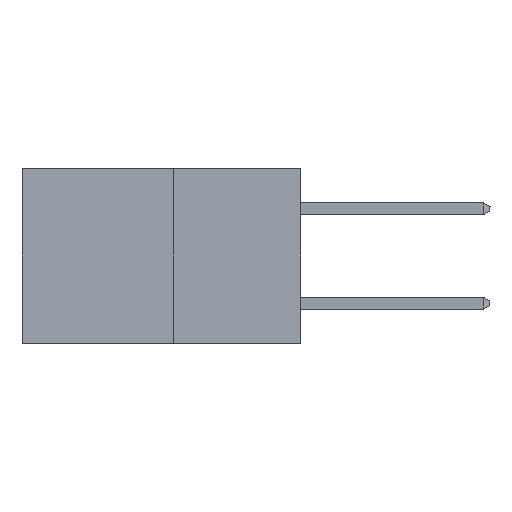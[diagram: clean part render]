
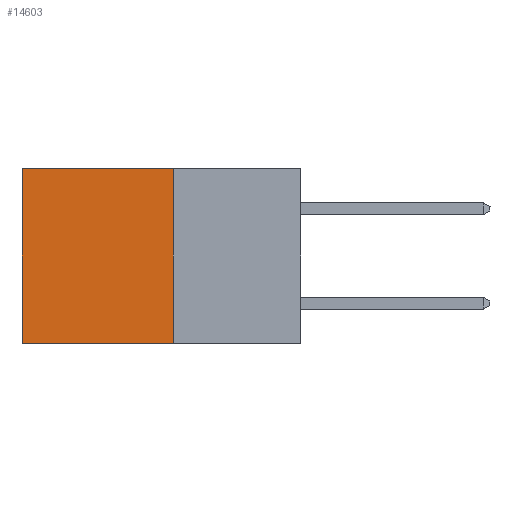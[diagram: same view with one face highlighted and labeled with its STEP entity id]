
A CAD part, left-side view. The second image highlights one B-rep face of the part: STEP entity #14603.
In plain terms, the highlighted planar face has unit normal (-1, 0, 0).
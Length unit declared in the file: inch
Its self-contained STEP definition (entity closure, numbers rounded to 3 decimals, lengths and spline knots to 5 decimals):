
#872 = CARTESIAN_POINT ( 'NONE',  ( 0.277, 0.27, 0. ) ) ;
#960 = VERTEX_POINT ( 'NONE', #5564 ) ;
#1803 = VERTEX_POINT ( 'NONE', #12594 ) ;
#2059 = CARTESIAN_POINT ( 'NONE',  ( 0.277, 0.59, -0.37 ) ) ;
#3305 = AXIS2_PLACEMENT_3D ( 'NONE', #14105, #4311, #14167 ) ;
#3553 = DIRECTION ( 'NONE',  ( 0., 0., -1. ) ) ;
#4311 = DIRECTION ( 'NONE',  ( 1., 0., 0. ) ) ;
#4386 = VECTOR ( 'NONE', #3553, 39.37008 ) ;
#4569 = EDGE_CURVE ( 'NONE', #16371, #11281, #10069, .T. ) ;
#5119 = DIRECTION ( 'NONE',  ( 0., 1., 0. ) ) ;
#5558 = ORIENTED_EDGE ( 'NONE', *, *, #14233, .F. ) ;
#5564 = CARTESIAN_POINT ( 'NONE',  ( 0.277, 0.27, -0.37 ) ) ;
#5967 = CARTESIAN_POINT ( 'NONE',  ( 0.277, 0.27, 0. ) ) ;
#6186 = DIRECTION ( 'NONE',  ( 0., 1., 0. ) ) ;
#6847 = VECTOR ( 'NONE', #5119, 39.37008 ) ;
#6970 = CARTESIAN_POINT ( 'NONE',  ( 0.277, 0.59, 0. ) ) ;
#7265 = LINE ( 'NONE', #16370, #6847 ) ;
#7583 = DIRECTION ( 'NONE',  ( 0., 0., -1. ) ) ;
#7658 = EDGE_CURVE ( 'NONE', #960, #1803, #7265, .T. ) ;
#8397 = ORIENTED_EDGE ( 'NONE', *, *, #7658, .F. ) ;
#8823 = EDGE_CURVE ( 'NONE', #11281, #1803, #17061, .T. ) ;
#9875 = PLANE ( 'NONE',  #3305 ) ;
#10009 = VECTOR ( 'NONE', #7583, 39.37008 ) ;
#10069 = LINE ( 'NONE', #5967, #10524 ) ;
#10169 = ORIENTED_EDGE ( 'NONE', *, *, #4569, .T. ) ;
#10524 = VECTOR ( 'NONE', #6186, 39.37008 ) ;
#11281 = VERTEX_POINT ( 'NONE', #6970 ) ;
#11404 = LINE ( 'NONE', #11930, #4386 ) ;
#11709 = ORIENTED_EDGE ( 'NONE', *, *, #8823, .T. ) ;
#11930 = CARTESIAN_POINT ( 'NONE',  ( 0.277, 0.27, -0.37 ) ) ;
#12594 = CARTESIAN_POINT ( 'NONE',  ( 0.277, 0.59, -0.37 ) ) ;
#14105 = CARTESIAN_POINT ( 'NONE',  ( 0.277, 0.27, -0.37 ) ) ;
#14167 = DIRECTION ( 'NONE',  ( 0., 0., -1. ) ) ;
#14233 = EDGE_CURVE ( 'NONE', #16371, #960, #11404, .T. ) ;
#14603 = ADVANCED_FACE ( 'NONE', ( #14944 ), #9875, .F. ) ;
#14944 = FACE_OUTER_BOUND ( 'NONE', #17531, .T. ) ;
#16370 = CARTESIAN_POINT ( 'NONE',  ( 0.277, 0.27, -0.37 ) ) ;
#16371 = VERTEX_POINT ( 'NONE', #872 ) ;
#17061 = LINE ( 'NONE', #2059, #10009 ) ;
#17531 = EDGE_LOOP ( 'NONE', ( #11709, #8397, #5558, #10169 ) ) ;
